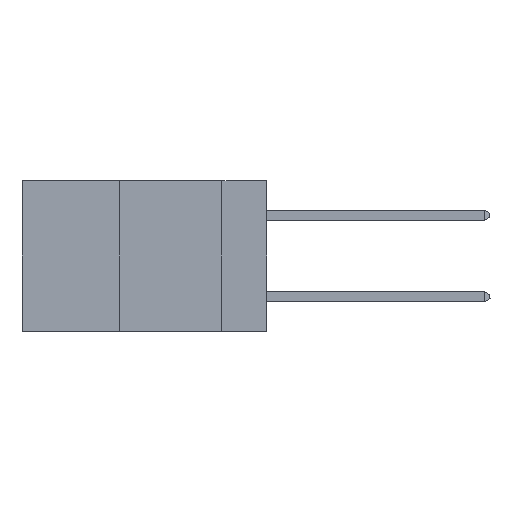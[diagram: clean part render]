
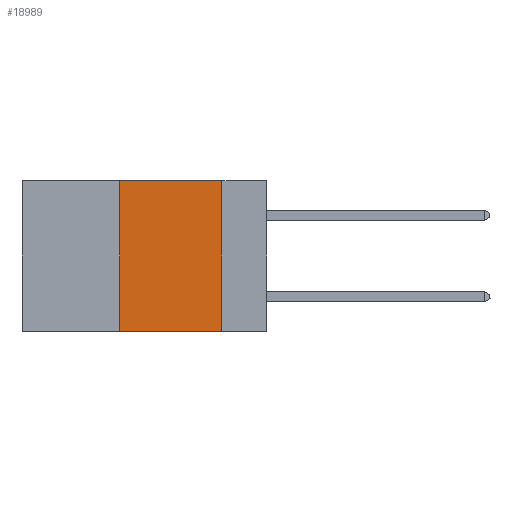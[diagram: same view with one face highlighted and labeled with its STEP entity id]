
A CAD part, left-side view. The second image highlights one B-rep face of the part: STEP entity #18989.
In plain terms, the highlighted planar face has unit normal (-1, 0, 0).
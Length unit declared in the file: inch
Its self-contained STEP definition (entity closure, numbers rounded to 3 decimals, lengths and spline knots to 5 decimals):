
#113 = VECTOR ( 'NONE', #13916, 39.37008 ) ;
#643 = VERTEX_POINT ( 'NONE', #11509 ) ;
#1205 = CARTESIAN_POINT ( 'NONE',  ( 0., 0.11, 0. ) ) ;
#2129 = DIRECTION ( 'NONE',  ( 0., -1., 0. ) ) ;
#2155 = VERTEX_POINT ( 'NONE', #15876 ) ;
#3377 = AXIS2_PLACEMENT_3D ( 'NONE', #18358, #11491, #18737 ) ;
#4653 = LINE ( 'NONE', #22336, #5461 ) ;
#4716 = VECTOR ( 'NONE', #7788, 39.37008 ) ;
#5461 = VECTOR ( 'NONE', #18782, 39.37008 ) ;
#5471 = CARTESIAN_POINT ( 'NONE',  ( 0., 0.11, 0. ) ) ;
#5731 = CARTESIAN_POINT ( 'NONE',  ( 0., 0.6, -0.37 ) ) ;
#6081 = ORIENTED_EDGE ( 'NONE', *, *, #21595, .T. ) ;
#6841 = EDGE_LOOP ( 'NONE', ( #9400, #19080, #18808, #6081 ) ) ;
#7694 = PLANE ( 'NONE',  #3377 ) ;
#7788 = DIRECTION ( 'NONE',  ( 0., 0., -1. ) ) ;
#8018 = LINE ( 'NONE', #5471, #4716 ) ;
#8477 = CARTESIAN_POINT ( 'NONE',  ( 0., 0.36, -0.37 ) ) ;
#9400 = ORIENTED_EDGE ( 'NONE', *, *, #16550, .F. ) ;
#9781 = EDGE_CURVE ( 'NONE', #643, #10176, #4653, .T. ) ;
#9939 = LINE ( 'NONE', #5731, #13495 ) ;
#10176 = VERTEX_POINT ( 'NONE', #1205 ) ;
#10533 = LINE ( 'NONE', #19195, #113 ) ;
#11167 = VERTEX_POINT ( 'NONE', #8477 ) ;
#11491 = DIRECTION ( 'NONE',  ( 1., 0., 0. ) ) ;
#11509 = CARTESIAN_POINT ( 'NONE',  ( 0., 0.36, 0. ) ) ;
#13495 = VECTOR ( 'NONE', #2129, 39.37008 ) ;
#13916 = DIRECTION ( 'NONE',  ( 0., 0., 1. ) ) ;
#15876 = CARTESIAN_POINT ( 'NONE',  ( 0., 0.11, -0.37 ) ) ;
#16550 = EDGE_CURVE ( 'NONE', #10176, #2155, #8018, .T. ) ;
#18358 = CARTESIAN_POINT ( 'NONE',  ( 0., 0.6, 0. ) ) ;
#18737 = DIRECTION ( 'NONE',  ( 0., 0., -1. ) ) ;
#18782 = DIRECTION ( 'NONE',  ( 0., -1., 0. ) ) ;
#18808 = ORIENTED_EDGE ( 'NONE', *, *, #20266, .F. ) ;
#18989 = ADVANCED_FACE ( 'NONE', ( #21342 ), #7694, .F. ) ;
#19080 = ORIENTED_EDGE ( 'NONE', *, *, #9781, .F. ) ;
#19195 = CARTESIAN_POINT ( 'NONE',  ( 0., 0.36, 0. ) ) ;
#20266 = EDGE_CURVE ( 'NONE', #11167, #643, #10533, .T. ) ;
#21342 = FACE_OUTER_BOUND ( 'NONE', #6841, .T. ) ;
#21595 = EDGE_CURVE ( 'NONE', #11167, #2155, #9939, .T. ) ;
#22336 = CARTESIAN_POINT ( 'NONE',  ( 0., 0.6, 0. ) ) ;
